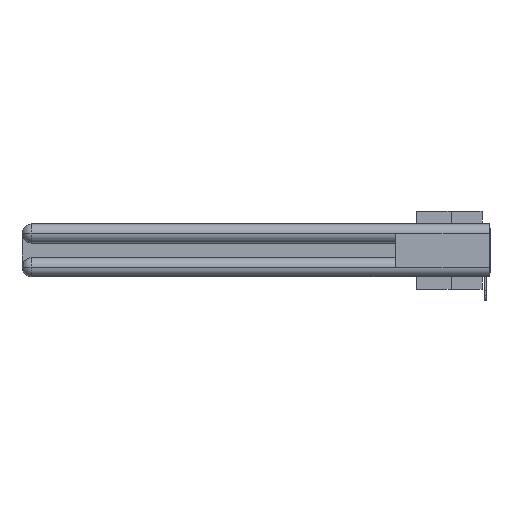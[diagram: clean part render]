
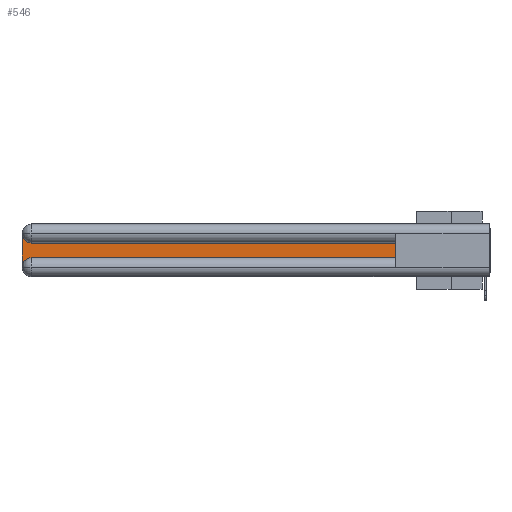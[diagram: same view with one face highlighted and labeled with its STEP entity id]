
A CAD part, left-side view. The second image highlights one B-rep face of the part: STEP entity #546.
In plain terms, the highlighted planar face has unit normal (-1, 0, 0).
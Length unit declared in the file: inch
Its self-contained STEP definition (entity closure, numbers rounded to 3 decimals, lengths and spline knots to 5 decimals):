
#255 = PLANE ( 'NONE',  #7600 ) ;
#546 = ADVANCED_FACE ( 'NONE', ( #10869 ), #255, .F. ) ;
#756 = CARTESIAN_POINT ( 'NONE',  ( 0.075, 2.94, -0.1225 ) ) ;
#2452 = LINE ( 'NONE', #26934, #14908 ) ;
#2602 = EDGE_CURVE ( 'NONE', #9348, #22722, #6953, .T. ) ;
#2733 = ORIENTED_EDGE ( 'NONE', *, *, #2602, .T. ) ;
#3591 = LINE ( 'NONE', #15841, #13727 ) ;
#3917 = ORIENTED_EDGE ( 'NONE', *, *, #16262, .T. ) ;
#4051 = DIRECTION ( 'NONE',  ( 0., -1., 0. ) ) ;
#5416 = EDGE_CURVE ( 'NONE', #7504, #8503, #19815, .T. ) ;
#6099 = CARTESIAN_POINT ( 'NONE',  ( 0.075, 0.6, -0.2175 ) ) ;
#6516 = CARTESIAN_POINT ( 'NONE',  ( 0.075, 2.94, -0.2775 ) ) ;
#6953 = LINE ( 'NONE', #25514, #19467 ) ;
#7504 = VERTEX_POINT ( 'NONE', #756 ) ;
#7600 = AXIS2_PLACEMENT_3D ( 'NONE', #10267, #22887, #14958 ) ;
#8503 = VERTEX_POINT ( 'NONE', #28892 ) ;
#9244 = CARTESIAN_POINT ( 'NONE',  ( 0.075, 3., -0.2775 ) ) ;
#9348 = VERTEX_POINT ( 'NONE', #30041 ) ;
#10267 = CARTESIAN_POINT ( 'NONE',  ( 0.075, 3., -0.1225 ) ) ;
#10869 = FACE_OUTER_BOUND ( 'NONE', #28919, .T. ) ;
#12890 = VERTEX_POINT ( 'NONE', #9244 ) ;
#12924 = EDGE_CURVE ( 'NONE', #8503, #12890, #2452, .T. ) ;
#13371 = DIRECTION ( 'NONE',  ( 0., 1., 0. ) ) ;
#13727 = VECTOR ( 'NONE', #13371, 39.37008 ) ;
#14174 = DIRECTION ( 'NONE',  ( 1., 0., 0. ) ) ;
#14883 = CIRCLE ( 'NONE', #30877, 0.06 ) ;
#14908 = VECTOR ( 'NONE', #31730, 39.37008 ) ;
#14958 = DIRECTION ( 'NONE',  ( 0., 0., -1. ) ) ;
#15841 = CARTESIAN_POINT ( 'NONE',  ( 0.075, 0.6, -0.1225 ) ) ;
#16262 = EDGE_CURVE ( 'NONE', #20350, #9348, #29013, .T. ) ;
#16369 = ORIENTED_EDGE ( 'NONE', *, *, #17539, .T. ) ;
#16450 = CARTESIAN_POINT ( 'NONE',  ( 0.075, 2.94, -0.0625 ) ) ;
#16473 = DIRECTION ( 'NONE',  ( 0., 0., -1. ) ) ;
#17539 = EDGE_CURVE ( 'NONE', #22722, #7504, #3591, .T. ) ;
#17729 = VECTOR ( 'NONE', #4051, 39.37008 ) ;
#18860 = DIRECTION ( 'NONE',  ( 0., 0., -1. ) ) ;
#19467 = VECTOR ( 'NONE', #23314, 39.37008 ) ;
#19608 = CARTESIAN_POINT ( 'NONE',  ( 0.075, 2.94, -0.2175 ) ) ;
#19815 = CIRCLE ( 'NONE', #28801, 0.06 ) ;
#20313 = ORIENTED_EDGE ( 'NONE', *, *, #12924, .T. ) ;
#20350 = VERTEX_POINT ( 'NONE', #19608 ) ;
#21846 = ORIENTED_EDGE ( 'NONE', *, *, #5416, .T. ) ;
#22722 = VERTEX_POINT ( 'NONE', #29432 ) ;
#22887 = DIRECTION ( 'NONE',  ( 1., 0., 0. ) ) ;
#23114 = ORIENTED_EDGE ( 'NONE', *, *, #31067, .T. ) ;
#23314 = DIRECTION ( 'NONE',  ( 0., 0., 1. ) ) ;
#24074 = DIRECTION ( 'NONE',  ( 1., 0., 0. ) ) ;
#25514 = CARTESIAN_POINT ( 'NONE',  ( 0.075, 0.6, -0.2175 ) ) ;
#26934 = CARTESIAN_POINT ( 'NONE',  ( 0.075, 3., -0.2175 ) ) ;
#28801 = AXIS2_PLACEMENT_3D ( 'NONE', #16450, #14174, #18860 ) ;
#28892 = CARTESIAN_POINT ( 'NONE',  ( 0.075, 3., -0.0625 ) ) ;
#28919 = EDGE_LOOP ( 'NONE', ( #16369, #21846, #20313, #23114, #3917, #2733 ) ) ;
#29013 = LINE ( 'NONE', #6099, #17729 ) ;
#29432 = CARTESIAN_POINT ( 'NONE',  ( 0.075, 0.6, -0.1225 ) ) ;
#30041 = CARTESIAN_POINT ( 'NONE',  ( 0.075, 0.6, -0.2175 ) ) ;
#30877 = AXIS2_PLACEMENT_3D ( 'NONE', #6516, #24074, #16473 ) ;
#31067 = EDGE_CURVE ( 'NONE', #12890, #20350, #14883, .T. ) ;
#31730 = DIRECTION ( 'NONE',  ( 0., 0., -1. ) ) ;
